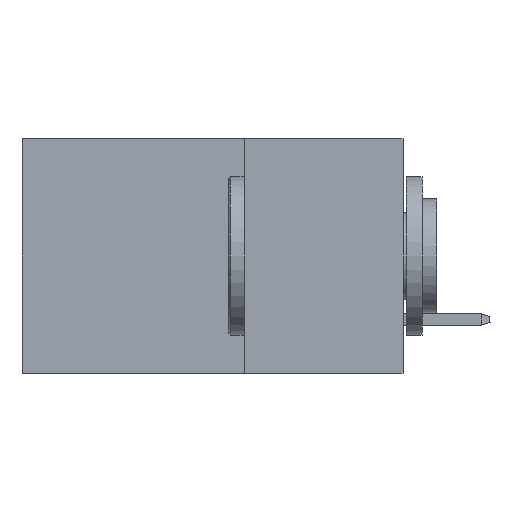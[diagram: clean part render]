
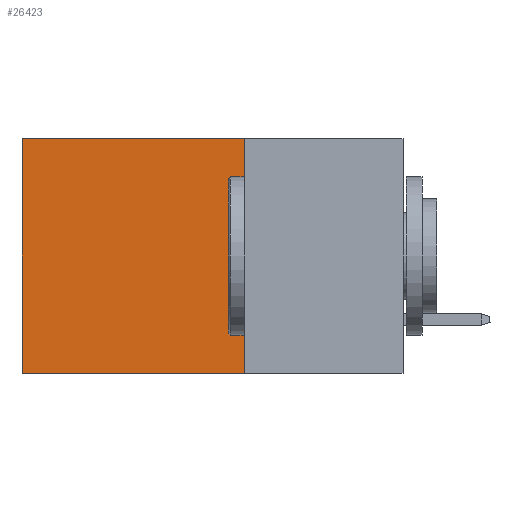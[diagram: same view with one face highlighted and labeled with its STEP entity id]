
A CAD part, left-side view. The second image highlights one B-rep face of the part: STEP entity #26423.
In plain terms, the highlighted planar face has unit normal (-1, 0, 0).
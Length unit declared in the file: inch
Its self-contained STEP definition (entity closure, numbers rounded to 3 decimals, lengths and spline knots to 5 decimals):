
#399 = CARTESIAN_POINT ( 'NONE',  ( 0.2875, 0.25, -0.37 ) ) ;
#1861 = ORIENTED_EDGE ( 'NONE', *, *, #42234, .F. ) ;
#3083 = ORIENTED_EDGE ( 'NONE', *, *, #21894, .F. ) ;
#10041 = DIRECTION ( 'NONE',  ( 0., 1., 0. ) ) ;
#10609 = CARTESIAN_POINT ( 'NONE',  ( 0.2875, 0.25, -0.37 ) ) ;
#11145 = VECTOR ( 'NONE', #10041, 39.37008 ) ;
#12264 = VERTEX_POINT ( 'NONE', #32938 ) ;
#12695 = EDGE_CURVE ( 'NONE', #30080, #40112, #28907, .T. ) ;
#13086 = VECTOR ( 'NONE', #37850, 39.37008 ) ;
#15706 = LINE ( 'NONE', #44160, #30599 ) ;
#15957 = AXIS2_PLACEMENT_3D ( 'NONE', #27452, #44900, #23511 ) ;
#17947 = VERTEX_POINT ( 'NONE', #10609 ) ;
#21894 = EDGE_CURVE ( 'NONE', #17947, #12264, #30287, .T. ) ;
#22380 = FACE_OUTER_BOUND ( 'NONE', #35306, .T. ) ;
#23511 = DIRECTION ( 'NONE',  ( 0., 0., -1. ) ) ;
#25439 = VECTOR ( 'NONE', #29272, 39.37008 ) ;
#26423 = ADVANCED_FACE ( 'NONE', ( #22380 ), #40982, .F. ) ;
#27452 = CARTESIAN_POINT ( 'NONE',  ( 0.2875, 0.25, 0. ) ) ;
#28403 = CARTESIAN_POINT ( 'NONE',  ( 0.2875, 0.25, 0. ) ) ;
#28907 = LINE ( 'NONE', #44064, #11145 ) ;
#29272 = DIRECTION ( 'NONE',  ( 0., 0., -1. ) ) ;
#30080 = VERTEX_POINT ( 'NONE', #28403 ) ;
#30287 = LINE ( 'NONE', #399, #13086 ) ;
#30599 = VECTOR ( 'NONE', #40739, 39.37008 ) ;
#32938 = CARTESIAN_POINT ( 'NONE',  ( 0.2875, 0.6, -0.37 ) ) ;
#35306 = EDGE_LOOP ( 'NONE', ( #44641, #3083, #1861, #45257 ) ) ;
#36050 = EDGE_CURVE ( 'NONE', #40112, #12264, #15706, .T. ) ;
#37584 = LINE ( 'NONE', #44194, #25439 ) ;
#37850 = DIRECTION ( 'NONE',  ( 0., 1., 0. ) ) ;
#40112 = VERTEX_POINT ( 'NONE', #45046 ) ;
#40739 = DIRECTION ( 'NONE',  ( 0., 0., -1. ) ) ;
#40982 = PLANE ( 'NONE',  #15957 ) ;
#42234 = EDGE_CURVE ( 'NONE', #30080, #17947, #37584, .T. ) ;
#44064 = CARTESIAN_POINT ( 'NONE',  ( 0.2875, 0.25, 0. ) ) ;
#44160 = CARTESIAN_POINT ( 'NONE',  ( 0.2875, 0.6, 0. ) ) ;
#44194 = CARTESIAN_POINT ( 'NONE',  ( 0.2875, 0.25, 0. ) ) ;
#44641 = ORIENTED_EDGE ( 'NONE', *, *, #36050, .T. ) ;
#44900 = DIRECTION ( 'NONE',  ( 1., 0., 0. ) ) ;
#45046 = CARTESIAN_POINT ( 'NONE',  ( 0.2875, 0.6, 0. ) ) ;
#45257 = ORIENTED_EDGE ( 'NONE', *, *, #12695, .T. ) ;
